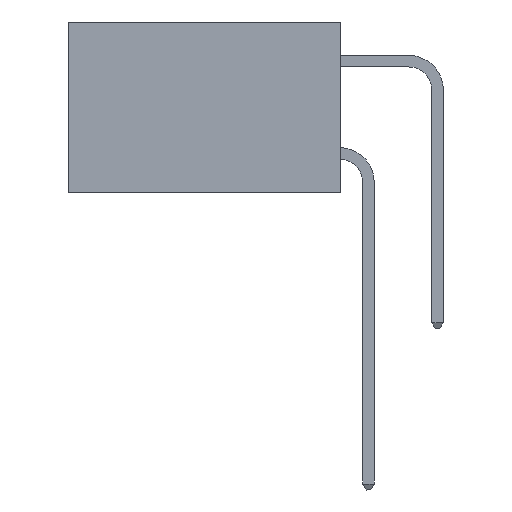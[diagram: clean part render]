
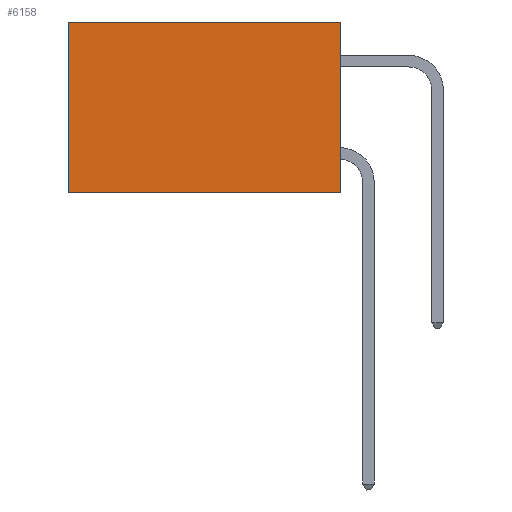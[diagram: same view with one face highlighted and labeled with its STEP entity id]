
A CAD part, left-side view. The second image highlights one B-rep face of the part: STEP entity #6158.
In plain terms, the highlighted planar face has unit normal (-1, 0, 0).
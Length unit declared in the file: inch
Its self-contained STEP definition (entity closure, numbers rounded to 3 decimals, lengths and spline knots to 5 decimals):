
#115 = CARTESIAN_POINT ( 'NONE',  ( 0.277, 0., -0.37 ) ) ;
#192 = EDGE_CURVE ( 'NONE', #3951, #7646, #8967, .T. ) ;
#1265 = CARTESIAN_POINT ( 'NONE',  ( 0.277, 0.59, -0.37 ) ) ;
#1577 = EDGE_LOOP ( 'NONE', ( #6218, #6120, #7594, #6336 ) ) ;
#1600 = LINE ( 'NONE', #6342, #7093 ) ;
#1611 = VECTOR ( 'NONE', #3463, 39.37008 ) ;
#2061 = LINE ( 'NONE', #3796, #1611 ) ;
#2920 = EDGE_CURVE ( 'NONE', #7646, #6474, #2061, .T. ) ;
#3065 = VERTEX_POINT ( 'NONE', #115 ) ;
#3103 = CARTESIAN_POINT ( 'NONE',  ( 0.277, 0., -0.37 ) ) ;
#3296 = EDGE_CURVE ( 'NONE', #3065, #6474, #1600, .T. ) ;
#3463 = DIRECTION ( 'NONE',  ( 0., 0., -1. ) ) ;
#3780 = DIRECTION ( 'NONE',  ( 1., 0., 0. ) ) ;
#3796 = CARTESIAN_POINT ( 'NONE',  ( 0.277, 0.59, -0.37 ) ) ;
#3951 = VERTEX_POINT ( 'NONE', #8873 ) ;
#4098 = CARTESIAN_POINT ( 'NONE',  ( 0.277, 0., -0.37 ) ) ;
#4124 = DIRECTION ( 'NONE',  ( 0., 0., -1. ) ) ;
#4562 = CARTESIAN_POINT ( 'NONE',  ( 0.277, 0.59, 0. ) ) ;
#4673 = DIRECTION ( 'NONE',  ( 0., 1., 0. ) ) ;
#5490 = DIRECTION ( 'NONE',  ( 0., 1., 0. ) ) ;
#6120 = ORIENTED_EDGE ( 'NONE', *, *, #3296, .F. ) ;
#6158 = ADVANCED_FACE ( 'NONE', ( #6464 ), #7404, .F. ) ;
#6218 = ORIENTED_EDGE ( 'NONE', *, *, #2920, .T. ) ;
#6336 = ORIENTED_EDGE ( 'NONE', *, *, #192, .T. ) ;
#6342 = CARTESIAN_POINT ( 'NONE',  ( 0.277, 0., -0.37 ) ) ;
#6464 = FACE_OUTER_BOUND ( 'NONE', #1577, .T. ) ;
#6474 = VERTEX_POINT ( 'NONE', #1265 ) ;
#7093 = VECTOR ( 'NONE', #5490, 39.37008 ) ;
#7187 = VECTOR ( 'NONE', #4673, 39.37008 ) ;
#7222 = CARTESIAN_POINT ( 'NONE',  ( 0.277, 0., 0. ) ) ;
#7261 = EDGE_CURVE ( 'NONE', #3951, #3065, #7291, .T. ) ;
#7291 = LINE ( 'NONE', #4098, #8456 ) ;
#7404 = PLANE ( 'NONE',  #9158 ) ;
#7594 = ORIENTED_EDGE ( 'NONE', *, *, #7261, .F. ) ;
#7646 = VERTEX_POINT ( 'NONE', #4562 ) ;
#8456 = VECTOR ( 'NONE', #4124, 39.37008 ) ;
#8761 = DIRECTION ( 'NONE',  ( 0., 0., -1. ) ) ;
#8873 = CARTESIAN_POINT ( 'NONE',  ( 0.277, 0., 0. ) ) ;
#8967 = LINE ( 'NONE', #7222, #7187 ) ;
#9158 = AXIS2_PLACEMENT_3D ( 'NONE', #3103, #3780, #8761 ) ;
